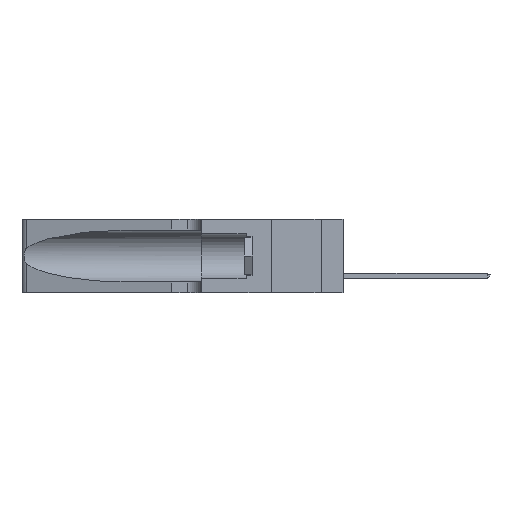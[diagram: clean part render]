
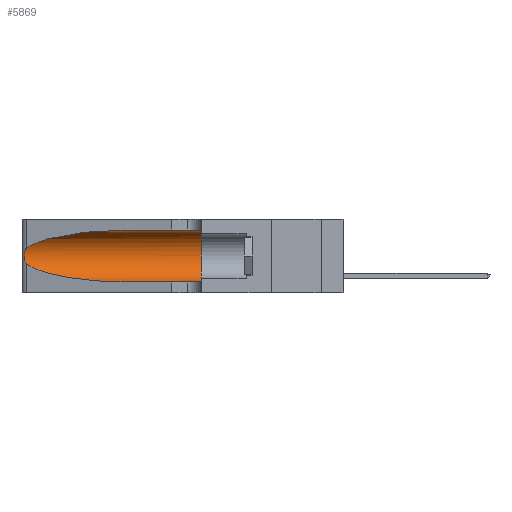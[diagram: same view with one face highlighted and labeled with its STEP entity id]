
A CAD part, left-side view. The second image highlights one B-rep face of the part: STEP entity #5869.
In plain terms, the highlighted cylindrical face has radius 3.308 mm (diameter 6.617 mm), a partial arc.
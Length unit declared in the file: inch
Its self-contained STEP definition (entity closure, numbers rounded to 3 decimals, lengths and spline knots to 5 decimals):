
#137 = EDGE_CURVE ( 'NONE', #30563, #16993, #7700, .T. ) ;
#1793 =( BOUNDED_CURVE ( )  B_SPLINE_CURVE ( 3, ( #6956, #9544, #26975, #32552 ),
 .UNSPECIFIED., .F., .F. ) 
 B_SPLINE_CURVE_WITH_KNOTS ( ( 4, 4 ),
 ( 3.44316, 4.71239 ),
 .UNSPECIFIED. ) 
 CURVE ( )  GEOMETRIC_REPRESENTATION_ITEM ( )  RATIONAL_B_SPLINE_CURVE ( ( 1., 0.87, 0.87, 1. ) ) 
 REPRESENTATION_ITEM ( '' )  );
#2270 = LINE ( 'NONE', #5647, #19108 ) ;
#2390 = CARTESIAN_POINT ( 'NONE',  ( 0.25487, 1.22718, 0.22369 ) ) ;
#2420 = ORIENTED_EDGE ( 'NONE', *, *, #32513, .T. ) ;
#5177 = CARTESIAN_POINT ( 'NONE',  ( 0.25856, 1.23593, 0.16098 ) ) ;
#5502 = LINE ( 'NONE', #21509, #23946 ) ;
#5647 = CARTESIAN_POINT ( 'NONE',  ( 0.1305, 1.61858, 0.31525 ) ) ;
#5657 = B_SPLINE_CURVE_WITH_KNOTS ( 'NONE', 3,
 ( #7315, #15044, #30321, #32907, #22241, #6889, #24787, #9472, #27341, #5177, #7536, #22975, #30766, #30431 ),
 .UNSPECIFIED., .F., .F.,
 ( 4, 2, 2, 2, 2, 2, 4 ),
 ( 0., 0.00027, 0.00053, 0.00107, 0.0016, 0.00187, 0.00214 ),
 .UNSPECIFIED. ) ;
#5869 = ADVANCED_FACE ( 'NONE', ( #27034 ), #14657, .F. ) ;
#5898 = CIRCLE ( 'NONE', #22289, 0.13025 ) ;
#6317 = VERTEX_POINT ( 'NONE', #31249 ) ;
#6889 = CARTESIAN_POINT ( 'NONE',  ( 0.26018, 1.23835, 0.19895 ) ) ;
#6956 = CARTESIAN_POINT ( 'NONE',  ( 0.25487, 1.22718, 0.14631 ) ) ;
#7123 = EDGE_LOOP ( 'NONE', ( #22532, #2420, #26056, #25170, #31867, #32755 ) ) ;
#7315 = CARTESIAN_POINT ( 'NONE',  ( 0.25487, 1.22718, 0.22369 ) ) ;
#7536 = CARTESIAN_POINT ( 'NONE',  ( 0.25789, 1.23486, 0.15765 ) ) ;
#7648 = DIRECTION ( 'NONE',  ( 0., 1., 0. ) ) ;
#7700 =( BOUNDED_CURVE ( )  B_SPLINE_CURVE ( 3, ( #14162, #29536, #26986, #29755 ),
 .UNSPECIFIED., .F., .F. ) 
 B_SPLINE_CURVE_WITH_KNOTS ( ( 4, 4 ),
 ( 1.5708, 2.84003 ),
 .UNSPECIFIED. ) 
 CURVE ( )  GEOMETRIC_REPRESENTATION_ITEM ( )  RATIONAL_B_SPLINE_CURVE ( ( 1., 0.87, 0.87, 1. ) ) 
 REPRESENTATION_ITEM ( '' )  );
#8158 = CARTESIAN_POINT ( 'NONE',  ( 0.1305, 1.61858, 0.185 ) ) ;
#8759 = EDGE_CURVE ( 'NONE', #9739, #6317, #5502, .T. ) ;
#9472 = CARTESIAN_POINT ( 'NONE',  ( 0.26075, 1.23896, 0.178 ) ) ;
#9544 = CARTESIAN_POINT ( 'NONE',  ( 0.2373, 1.15595, 0.08982 ) ) ;
#9739 = VERTEX_POINT ( 'NONE', #13384 ) ;
#10228 = DIRECTION ( 'NONE',  ( 0., 0., 1. ) ) ;
#11649 = VERTEX_POINT ( 'NONE', #13150 ) ;
#13150 = CARTESIAN_POINT ( 'NONE',  ( 0.1305, 0.35, 0.31525 ) ) ;
#13384 = CARTESIAN_POINT ( 'NONE',  ( 0.1305, 0.72297, 0.05475 ) ) ;
#14162 = CARTESIAN_POINT ( 'NONE',  ( 0.1305, 0.72297, 0.31525 ) ) ;
#14657 = CYLINDRICAL_SURFACE ( 'NONE', #22463, 0.13025 ) ;
#15044 = CARTESIAN_POINT ( 'NONE',  ( 0.25555, 1.22994, 0.2215 ) ) ;
#15057 = EDGE_CURVE ( 'NONE', #19393, #9739, #1793, .T. ) ;
#16136 = DIRECTION ( 'NONE',  ( 0., -1., 0. ) ) ;
#16993 = VERTEX_POINT ( 'NONE', #2390 ) ;
#17435 = DIRECTION ( 'NONE',  ( 0., -1., 0. ) ) ;
#19108 = VECTOR ( 'NONE', #31358, 39.37008 ) ;
#19393 = VERTEX_POINT ( 'NONE', #22441 ) ;
#20102 = DIRECTION ( 'NONE',  ( 0., 0., -1. ) ) ;
#21509 = CARTESIAN_POINT ( 'NONE',  ( 0.1305, 1.61858, 0.05475 ) ) ;
#22241 = CARTESIAN_POINT ( 'NONE',  ( 0.25854, 1.2359, 0.20912 ) ) ;
#22289 = AXIS2_PLACEMENT_3D ( 'NONE', #25439, #7648, #10228 ) ;
#22441 = CARTESIAN_POINT ( 'NONE',  ( 0.25487, 1.22718, 0.14631 ) ) ;
#22463 = AXIS2_PLACEMENT_3D ( 'NONE', #8158, #17435, #20102 ) ;
#22532 = ORIENTED_EDGE ( 'NONE', *, *, #137, .T. ) ;
#22975 = CARTESIAN_POINT ( 'NONE',  ( 0.25639, 1.23186, 0.15144 ) ) ;
#23946 = VECTOR ( 'NONE', #16136, 39.37008 ) ;
#24787 = CARTESIAN_POINT ( 'NONE',  ( 0.26075, 1.23896, 0.19203 ) ) ;
#25170 = ORIENTED_EDGE ( 'NONE', *, *, #8759, .T. ) ;
#25439 = CARTESIAN_POINT ( 'NONE',  ( 0.1305, 0.35, 0.185 ) ) ;
#26056 = ORIENTED_EDGE ( 'NONE', *, *, #15057, .T. ) ;
#26975 = CARTESIAN_POINT ( 'NONE',  ( 0.18966, 0.96281, 0.05475 ) ) ;
#26986 = CARTESIAN_POINT ( 'NONE',  ( 0.2373, 1.15595, 0.28018 ) ) ;
#27034 = FACE_OUTER_BOUND ( 'NONE', #7123, .T. ) ;
#27341 = CARTESIAN_POINT ( 'NONE',  ( 0.26017, 1.23833, 0.17102 ) ) ;
#28361 = EDGE_CURVE ( 'NONE', #30563, #11649, #2270, .T. ) ;
#28833 = CARTESIAN_POINT ( 'NONE',  ( 0.1305, 0.72297, 0.31525 ) ) ;
#29536 = CARTESIAN_POINT ( 'NONE',  ( 0.18966, 0.96281, 0.31525 ) ) ;
#29755 = CARTESIAN_POINT ( 'NONE',  ( 0.25487, 1.22718, 0.22369 ) ) ;
#30321 = CARTESIAN_POINT ( 'NONE',  ( 0.25639, 1.23184, 0.21858 ) ) ;
#30431 = CARTESIAN_POINT ( 'NONE',  ( 0.25487, 1.22718, 0.14631 ) ) ;
#30563 = VERTEX_POINT ( 'NONE', #28833 ) ;
#30766 = CARTESIAN_POINT ( 'NONE',  ( 0.25555, 1.22993, 0.14849 ) ) ;
#31249 = CARTESIAN_POINT ( 'NONE',  ( 0.1305, 0.35, 0.05475 ) ) ;
#31358 = DIRECTION ( 'NONE',  ( 0., -1., 0. ) ) ;
#31867 = ORIENTED_EDGE ( 'NONE', *, *, #32573, .F. ) ;
#32513 = EDGE_CURVE ( 'NONE', #16993, #19393, #5657, .T. ) ;
#32552 = CARTESIAN_POINT ( 'NONE',  ( 0.1305, 0.72297, 0.05475 ) ) ;
#32573 = EDGE_CURVE ( 'NONE', #11649, #6317, #5898, .T. ) ;
#32755 = ORIENTED_EDGE ( 'NONE', *, *, #28361, .F. ) ;
#32907 = CARTESIAN_POINT ( 'NONE',  ( 0.25787, 1.23484, 0.2124 ) ) ;
